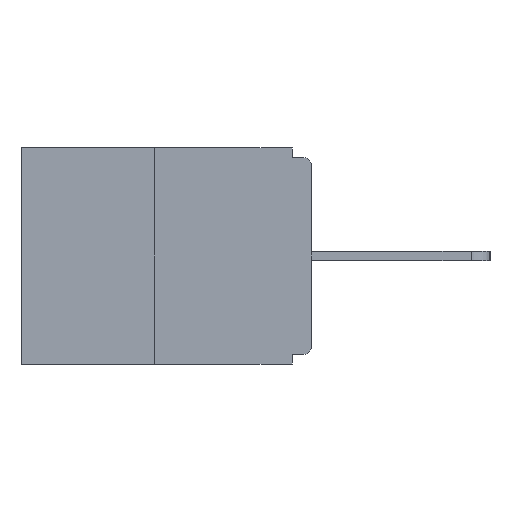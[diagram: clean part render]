
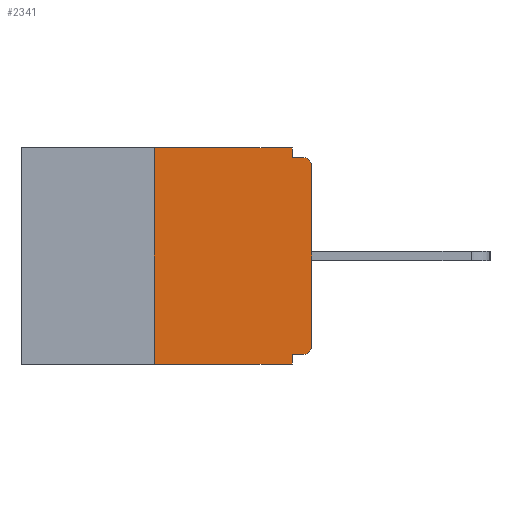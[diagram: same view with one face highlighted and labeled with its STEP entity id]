
A CAD part, left-side view. The second image highlights one B-rep face of the part: STEP entity #2341.
In plain terms, the highlighted planar face has unit normal (-1, 0, 0).
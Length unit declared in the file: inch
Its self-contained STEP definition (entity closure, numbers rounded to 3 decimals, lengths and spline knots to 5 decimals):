
#72 = VERTEX_POINT ( 'NONE', #12781 ) ;
#122 = CARTESIAN_POINT ( 'NONE',  ( 0., 0.015, -0.03 ) ) ;
#340 = CARTESIAN_POINT ( 'NONE',  ( 0., 0.015, -0.015 ) ) ;
#450 = CARTESIAN_POINT ( 'NONE',  ( 0., 0.031, -0.015 ) ) ;
#789 = CIRCLE ( 'NONE', #14241, 0.015 ) ;
#993 = LINE ( 'NONE', #9043, #7496 ) ;
#1380 = DIRECTION ( 'NONE',  ( 0., 1., 0. ) ) ;
#1476 = EDGE_CURVE ( 'NONE', #7429, #1566, #789, .T. ) ;
#1566 = VERTEX_POINT ( 'NONE', #340 ) ;
#1591 = EDGE_CURVE ( 'NONE', #5517, #3664, #14120, .T. ) ;
#1701 = DIRECTION ( 'NONE',  ( 0., 0., -1. ) ) ;
#1763 = EDGE_CURVE ( 'NONE', #72, #6849, #993, .T. ) ;
#1776 = DIRECTION ( 'NONE',  ( -1., 0., 0. ) ) ;
#1838 = CARTESIAN_POINT ( 'NONE',  ( 0., 0.015, -0.313 ) ) ;
#1854 = VERTEX_POINT ( 'NONE', #5134 ) ;
#1874 = LINE ( 'NONE', #3945, #13161 ) ;
#1983 = CARTESIAN_POINT ( 'NONE',  ( 0., 0.031, 0. ) ) ;
#2011 = EDGE_LOOP ( 'NONE', ( #4115, #4139, #4503, #4707, #5074, #5198, #5336, #5433, #5856, #5894 ) ) ;
#2096 = LINE ( 'NONE', #10317, #5154 ) ;
#2341 = ADVANCED_FACE ( 'NONE', ( #7648 ), #10950, .F. ) ;
#2383 = EDGE_CURVE ( 'NONE', #1854, #9950, #10457, .T. ) ;
#2429 = AXIS2_PLACEMENT_3D ( 'NONE', #1838, #1776, #1701 ) ;
#2558 = LINE ( 'NONE', #12985, #13810 ) ;
#2675 = DIRECTION ( 'NONE',  ( -1., 0., 0. ) ) ;
#2730 = DIRECTION ( 'NONE',  ( 0., 0., -1. ) ) ;
#3018 = AXIS2_PLACEMENT_3D ( 'NONE', #10324, #10308, #6925 ) ;
#3085 = LINE ( 'NONE', #4443, #14245 ) ;
#3161 = LINE ( 'NONE', #9039, #5816 ) ;
#3664 = VERTEX_POINT ( 'NONE', #4263 ) ;
#3945 = CARTESIAN_POINT ( 'NONE',  ( 0., 0., 0. ) ) ;
#4115 = ORIENTED_EDGE ( 'NONE', *, *, #1763, .F. ) ;
#4139 = ORIENTED_EDGE ( 'NONE', *, *, #9124, .F. ) ;
#4263 = CARTESIAN_POINT ( 'NONE',  ( 0., 0.031, -0.328 ) ) ;
#4315 = VECTOR ( 'NONE', #14350, 39.37008 ) ;
#4443 = CARTESIAN_POINT ( 'NONE',  ( 0., 0.031, -0.343 ) ) ;
#4495 = CARTESIAN_POINT ( 'NONE',  ( 0., 0.46, -0.343 ) ) ;
#4503 = ORIENTED_EDGE ( 'NONE', *, *, #2383, .T. ) ;
#4707 = ORIENTED_EDGE ( 'NONE', *, *, #12203, .F. ) ;
#5074 = ORIENTED_EDGE ( 'NONE', *, *, #1591, .F. ) ;
#5134 = CARTESIAN_POINT ( 'NONE',  ( 0., 0.25, -0.343 ) ) ;
#5154 = VECTOR ( 'NONE', #10282, 39.37008 ) ;
#5198 = ORIENTED_EDGE ( 'NONE', *, *, #7611, .T. ) ;
#5336 = ORIENTED_EDGE ( 'NONE', *, *, #14093, .T. ) ;
#5433 = ORIENTED_EDGE ( 'NONE', *, *, #1476, .T. ) ;
#5517 = VERTEX_POINT ( 'NONE', #10097 ) ;
#5816 = VECTOR ( 'NONE', #6910, 39.37008 ) ;
#5856 = ORIENTED_EDGE ( 'NONE', *, *, #10167, .F. ) ;
#5894 = ORIENTED_EDGE ( 'NONE', *, *, #7946, .F. ) ;
#6215 = CARTESIAN_POINT ( 'NONE',  ( 0., 0.031, -0.343 ) ) ;
#6849 = VERTEX_POINT ( 'NONE', #1983 ) ;
#6910 = DIRECTION ( 'NONE',  ( 0., 0., 1. ) ) ;
#6925 = DIRECTION ( 'NONE',  ( 0., 0., -1. ) ) ;
#7074 = CIRCLE ( 'NONE', #2429, 0.015 ) ;
#7429 = VERTEX_POINT ( 'NONE', #13236 ) ;
#7496 = VECTOR ( 'NONE', #9312, 39.37008 ) ;
#7611 = EDGE_CURVE ( 'NONE', #5517, #9763, #7074, .T. ) ;
#7648 = FACE_OUTER_BOUND ( 'NONE', #2011, .T. ) ;
#7946 = EDGE_CURVE ( 'NONE', #6849, #11523, #2096, .T. ) ;
#8428 = DIRECTION ( 'NONE',  ( 0., 0., 1. ) ) ;
#8503 = VECTOR ( 'NONE', #1380, 39.37008 ) ;
#8828 = DIRECTION ( 'NONE',  ( 0., -1., 0. ) ) ;
#9039 = CARTESIAN_POINT ( 'NONE',  ( 0., 0.25, 0. ) ) ;
#9043 = CARTESIAN_POINT ( 'NONE',  ( 0., 0.46, 0. ) ) ;
#9124 = EDGE_CURVE ( 'NONE', #1854, #72, #3161, .T. ) ;
#9312 = DIRECTION ( 'NONE',  ( 0., -1., 0. ) ) ;
#9763 = VERTEX_POINT ( 'NONE', #14359 ) ;
#9950 = VERTEX_POINT ( 'NONE', #6215 ) ;
#10097 = CARTESIAN_POINT ( 'NONE',  ( 0., 0.015, -0.328 ) ) ;
#10167 = EDGE_CURVE ( 'NONE', #11523, #1566, #2558, .T. ) ;
#10282 = DIRECTION ( 'NONE',  ( 0., 0., -1. ) ) ;
#10308 = DIRECTION ( 'NONE',  ( 1., 0., 0. ) ) ;
#10317 = CARTESIAN_POINT ( 'NONE',  ( 0., 0.031, 0. ) ) ;
#10324 = CARTESIAN_POINT ( 'NONE',  ( 0., 0.46, 0. ) ) ;
#10457 = LINE ( 'NONE', #4495, #4315 ) ;
#10683 = CARTESIAN_POINT ( 'NONE',  ( 0., 0., -0.328 ) ) ;
#10950 = PLANE ( 'NONE',  #3018 ) ;
#11523 = VERTEX_POINT ( 'NONE', #450 ) ;
#12004 = DIRECTION ( 'NONE',  ( 0., 0., -1. ) ) ;
#12203 = EDGE_CURVE ( 'NONE', #3664, #9950, #3085, .T. ) ;
#12781 = CARTESIAN_POINT ( 'NONE',  ( 0., 0.25, 0. ) ) ;
#12985 = CARTESIAN_POINT ( 'NONE',  ( 0., 0., -0.015 ) ) ;
#13161 = VECTOR ( 'NONE', #8428, 39.37008 ) ;
#13236 = CARTESIAN_POINT ( 'NONE',  ( 0., 0., -0.03 ) ) ;
#13810 = VECTOR ( 'NONE', #8828, 39.37008 ) ;
#14093 = EDGE_CURVE ( 'NONE', #9763, #7429, #1874, .T. ) ;
#14120 = LINE ( 'NONE', #10683, #8503 ) ;
#14241 = AXIS2_PLACEMENT_3D ( 'NONE', #122, #2675, #2730 ) ;
#14245 = VECTOR ( 'NONE', #12004, 39.37008 ) ;
#14350 = DIRECTION ( 'NONE',  ( 0., -1., 0. ) ) ;
#14359 = CARTESIAN_POINT ( 'NONE',  ( 0., 0., -0.313 ) ) ;
